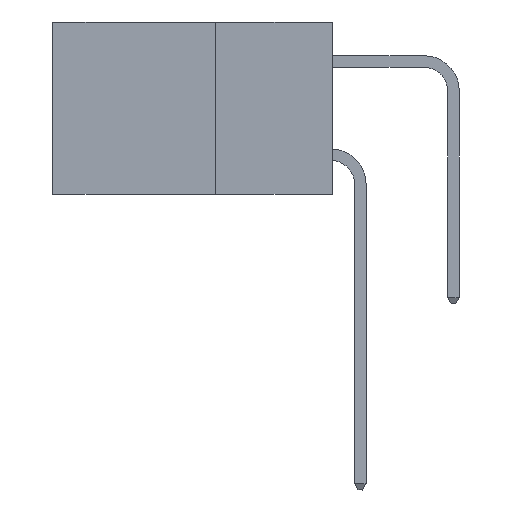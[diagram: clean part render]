
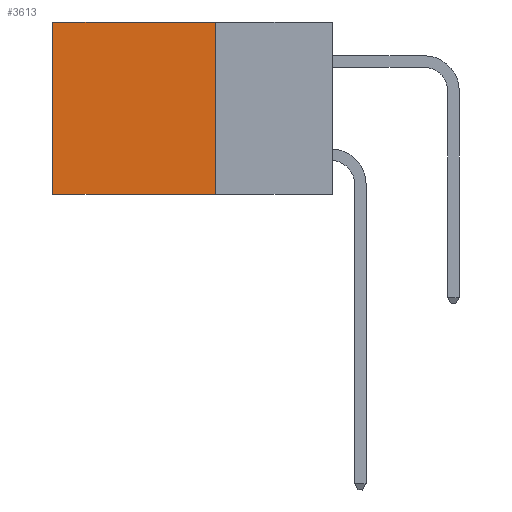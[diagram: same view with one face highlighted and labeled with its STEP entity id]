
A CAD part, left-side view. The second image highlights one B-rep face of the part: STEP entity #3613.
In plain terms, the highlighted planar face has unit normal (-1, 0, 0).
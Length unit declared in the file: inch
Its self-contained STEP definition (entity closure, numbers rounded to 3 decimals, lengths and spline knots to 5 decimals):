
#459 = DIRECTION ( 'NONE',  ( 1., 0., 0. ) ) ;
#1433 = DIRECTION ( 'NONE',  ( 0., 1., 0. ) ) ;
#1634 = VECTOR ( 'NONE', #1433, 39.37008 ) ;
#2039 = ORIENTED_EDGE ( 'NONE', *, *, #4789, .T. ) ;
#2629 = CARTESIAN_POINT ( 'NONE',  ( 0.298, 0.25, 0. ) ) ;
#3261 = EDGE_LOOP ( 'NONE', ( #2039, #8885, #16867, #3329 ) ) ;
#3329 = ORIENTED_EDGE ( 'NONE', *, *, #11997, .T. ) ;
#3613 = ADVANCED_FACE ( 'NONE', ( #7796 ), #15819, .F. ) ;
#4211 = LINE ( 'NONE', #2629, #12492 ) ;
#4636 = VERTEX_POINT ( 'NONE', #15078 ) ;
#4789 = EDGE_CURVE ( 'NONE', #12815, #19182, #18359, .T. ) ;
#4809 = LINE ( 'NONE', #6421, #5338 ) ;
#5338 = VECTOR ( 'NONE', #13551, 39.37008 ) ;
#6421 = CARTESIAN_POINT ( 'NONE',  ( 0.298, 0.25, -0.37 ) ) ;
#6895 = CARTESIAN_POINT ( 'NONE',  ( 0.298, 0.6, 0. ) ) ;
#7058 = CARTESIAN_POINT ( 'NONE',  ( 0.298, 0.25, 0. ) ) ;
#7796 = FACE_OUTER_BOUND ( 'NONE', #3261, .T. ) ;
#8126 = CARTESIAN_POINT ( 'NONE',  ( 0.298, 0.6, -0.37 ) ) ;
#8885 = ORIENTED_EDGE ( 'NONE', *, *, #17981, .F. ) ;
#9412 = DIRECTION ( 'NONE',  ( 0., 0., -1. ) ) ;
#9427 = VERTEX_POINT ( 'NONE', #14557 ) ;
#11997 = EDGE_CURVE ( 'NONE', #4636, #12815, #15545, .T. ) ;
#12492 = VECTOR ( 'NONE', #12863, 39.37008 ) ;
#12815 = VERTEX_POINT ( 'NONE', #6895 ) ;
#12863 = DIRECTION ( 'NONE',  ( 0., 0., -1. ) ) ;
#13044 = AXIS2_PLACEMENT_3D ( 'NONE', #7058, #459, #19040 ) ;
#13551 = DIRECTION ( 'NONE',  ( 0., 1., 0. ) ) ;
#14557 = CARTESIAN_POINT ( 'NONE',  ( 0.298, 0.25, -0.37 ) ) ;
#15078 = CARTESIAN_POINT ( 'NONE',  ( 0.298, 0.25, 0. ) ) ;
#15545 = LINE ( 'NONE', #20311, #1634 ) ;
#15819 = PLANE ( 'NONE',  #13044 ) ;
#16260 = CARTESIAN_POINT ( 'NONE',  ( 0.298, 0.6, 0. ) ) ;
#16867 = ORIENTED_EDGE ( 'NONE', *, *, #19073, .F. ) ;
#17981 = EDGE_CURVE ( 'NONE', #9427, #19182, #4809, .T. ) ;
#18359 = LINE ( 'NONE', #16260, #20748 ) ;
#19040 = DIRECTION ( 'NONE',  ( 0., 0., -1. ) ) ;
#19073 = EDGE_CURVE ( 'NONE', #4636, #9427, #4211, .T. ) ;
#19182 = VERTEX_POINT ( 'NONE', #8126 ) ;
#20311 = CARTESIAN_POINT ( 'NONE',  ( 0.298, 0.25, 0. ) ) ;
#20748 = VECTOR ( 'NONE', #9412, 39.37008 ) ;
